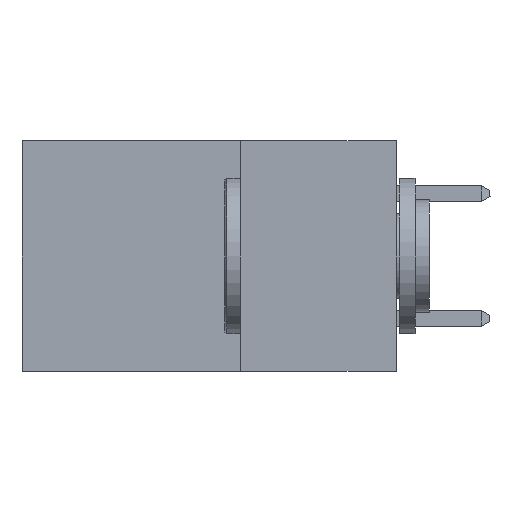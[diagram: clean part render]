
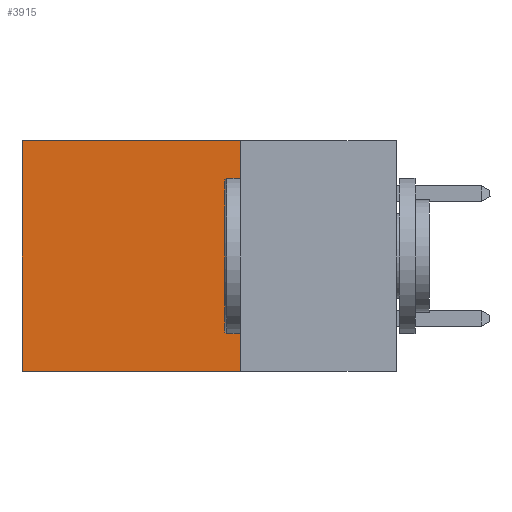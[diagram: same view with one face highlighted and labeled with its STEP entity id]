
A CAD part, left-side view. The second image highlights one B-rep face of the part: STEP entity #3915.
In plain terms, the highlighted planar face has unit normal (-1, 0, 0).
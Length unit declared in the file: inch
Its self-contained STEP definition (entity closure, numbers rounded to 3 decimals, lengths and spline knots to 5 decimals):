
#186 = EDGE_CURVE ( 'NONE', #10921, #18138, #11637, .T. ) ;
#470 = ORIENTED_EDGE ( 'NONE', *, *, #186, .T. ) ;
#622 = EDGE_LOOP ( 'NONE', ( #470, #9593, #12261, #5359 ) ) ;
#3555 = LINE ( 'NONE', #12183, #17181 ) ;
#3915 = ADVANCED_FACE ( 'NONE', ( #16687 ), #15008, .F. ) ;
#4618 = CARTESIAN_POINT ( 'NONE',  ( 0.2615, 0.25, 0. ) ) ;
#5359 = ORIENTED_EDGE ( 'NONE', *, *, #17081, .T. ) ;
#5580 = DIRECTION ( 'NONE',  ( 0., 0., -1. ) ) ;
#6600 = LINE ( 'NONE', #6745, #20647 ) ;
#6745 = CARTESIAN_POINT ( 'NONE',  ( 0.2615, 0.25, 0. ) ) ;
#7518 = CARTESIAN_POINT ( 'NONE',  ( 0.2615, 0.6, -0.37 ) ) ;
#8535 = DIRECTION ( 'NONE',  ( 0., 1., 0. ) ) ;
#9384 = DIRECTION ( 'NONE',  ( 0., 0., -1. ) ) ;
#9593 = ORIENTED_EDGE ( 'NONE', *, *, #14503, .F. ) ;
#9916 = EDGE_CURVE ( 'NONE', #17942, #16361, #16781, .T. ) ;
#10249 = CARTESIAN_POINT ( 'NONE',  ( 0.2615, 0.6, 0. ) ) ;
#10921 = VERTEX_POINT ( 'NONE', #10249 ) ;
#11637 = LINE ( 'NONE', #7518, #12203 ) ;
#12082 = VECTOR ( 'NONE', #9384, 39.37008 ) ;
#12179 = CARTESIAN_POINT ( 'NONE',  ( 0.2615, 0.6, -0.37 ) ) ;
#12183 = CARTESIAN_POINT ( 'NONE',  ( 0.2615, 0.25, -0.37 ) ) ;
#12203 = VECTOR ( 'NONE', #5580, 39.37008 ) ;
#12261 = ORIENTED_EDGE ( 'NONE', *, *, #9916, .F. ) ;
#14503 = EDGE_CURVE ( 'NONE', #16361, #18138, #3555, .T. ) ;
#14690 = CARTESIAN_POINT ( 'NONE',  ( 0.2615, 0.25, -0.37 ) ) ;
#14931 = DIRECTION ( 'NONE',  ( 0., 0., -1. ) ) ;
#14951 = DIRECTION ( 'NONE',  ( 1., 0., 0. ) ) ;
#14958 = CARTESIAN_POINT ( 'NONE',  ( 0.2615, 0.25, -0.37 ) ) ;
#15008 = PLANE ( 'NONE',  #21217 ) ;
#15476 = CARTESIAN_POINT ( 'NONE',  ( 0.2615, 0.25, -0.37 ) ) ;
#16361 = VERTEX_POINT ( 'NONE', #15476 ) ;
#16687 = FACE_OUTER_BOUND ( 'NONE', #622, .T. ) ;
#16781 = LINE ( 'NONE', #14690, #12082 ) ;
#17081 = EDGE_CURVE ( 'NONE', #17942, #10921, #6600, .T. ) ;
#17181 = VECTOR ( 'NONE', #19203, 39.37008 ) ;
#17942 = VERTEX_POINT ( 'NONE', #4618 ) ;
#18138 = VERTEX_POINT ( 'NONE', #12179 ) ;
#19203 = DIRECTION ( 'NONE',  ( 0., 1., 0. ) ) ;
#20647 = VECTOR ( 'NONE', #8535, 39.37008 ) ;
#21217 = AXIS2_PLACEMENT_3D ( 'NONE', #14958, #14951, #14931 ) ;
